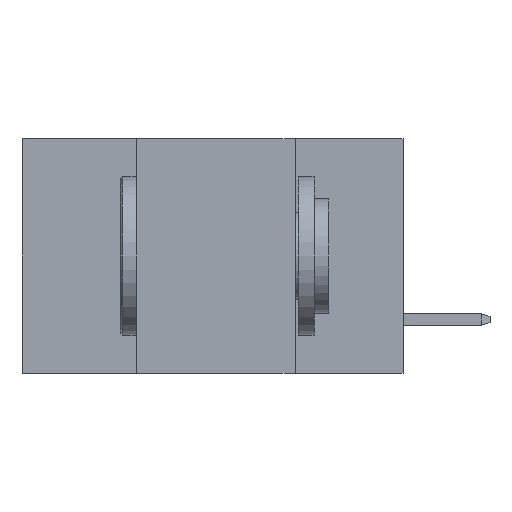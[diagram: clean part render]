
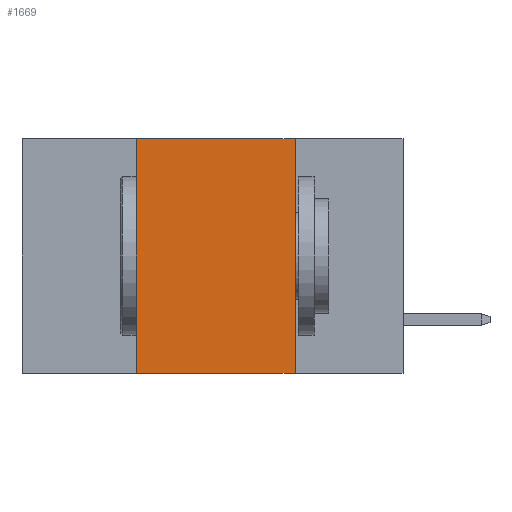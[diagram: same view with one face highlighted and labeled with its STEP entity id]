
A CAD part, left-side view. The second image highlights one B-rep face of the part: STEP entity #1669.
In plain terms, the highlighted planar face has unit normal (-1, 0, 0).
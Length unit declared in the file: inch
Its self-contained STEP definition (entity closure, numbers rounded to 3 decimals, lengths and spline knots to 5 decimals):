
#186 = AXIS2_PLACEMENT_3D ( 'NONE', #12351, #15154, #7084 ) ;
#1012 = ORIENTED_EDGE ( 'NONE', *, *, #2403, .F. ) ;
#1111 = EDGE_LOOP ( 'NONE', ( #17366, #12886, #1012, #2342 ) ) ;
#1669 = ADVANCED_FACE ( 'NONE', ( #16568 ), #1722, .F. ) ;
#1722 = PLANE ( 'NONE',  #186 ) ;
#1802 = CARTESIAN_POINT ( 'NONE',  ( 0., 0.42, 0. ) ) ;
#2342 = ORIENTED_EDGE ( 'NONE', *, *, #7177, .T. ) ;
#2403 = EDGE_CURVE ( 'NONE', #5977, #9764, #13399, .T. ) ;
#2577 = DIRECTION ( 'NONE',  ( 0., -1., 0. ) ) ;
#3229 = LINE ( 'NONE', #7332, #10016 ) ;
#3397 = VECTOR ( 'NONE', #6718, 39.37008 ) ;
#5225 = EDGE_CURVE ( 'NONE', #9764, #9868, #12114, .T. ) ;
#5361 = LINE ( 'NONE', #14443, #3397 ) ;
#5977 = VERTEX_POINT ( 'NONE', #16443 ) ;
#6151 = EDGE_CURVE ( 'NONE', #9868, #8075, #3229, .T. ) ;
#6718 = DIRECTION ( 'NONE',  ( 0., -1., 0. ) ) ;
#7084 = DIRECTION ( 'NONE',  ( 0., 0., -1. ) ) ;
#7177 = EDGE_CURVE ( 'NONE', #5977, #8075, #5361, .T. ) ;
#7332 = CARTESIAN_POINT ( 'NONE',  ( 0., 0.17, 0. ) ) ;
#7426 = DIRECTION ( 'NONE',  ( 0., 0., -1. ) ) ;
#7980 = VECTOR ( 'NONE', #2577, 39.37008 ) ;
#8075 = VERTEX_POINT ( 'NONE', #14685 ) ;
#9077 = CARTESIAN_POINT ( 'NONE',  ( 0., 0.17, 0. ) ) ;
#9764 = VERTEX_POINT ( 'NONE', #1802 ) ;
#9868 = VERTEX_POINT ( 'NONE', #9077 ) ;
#10016 = VECTOR ( 'NONE', #7426, 39.37008 ) ;
#12040 = VECTOR ( 'NONE', #13313, 39.37008 ) ;
#12114 = LINE ( 'NONE', #12391, #7980 ) ;
#12351 = CARTESIAN_POINT ( 'NONE',  ( 0., 0.6, 0. ) ) ;
#12391 = CARTESIAN_POINT ( 'NONE',  ( 0., 0.6, 0. ) ) ;
#12886 = ORIENTED_EDGE ( 'NONE', *, *, #5225, .F. ) ;
#13313 = DIRECTION ( 'NONE',  ( 0., 0., 1. ) ) ;
#13399 = LINE ( 'NONE', #14490, #12040 ) ;
#14443 = CARTESIAN_POINT ( 'NONE',  ( 0., 0.6, -0.37 ) ) ;
#14490 = CARTESIAN_POINT ( 'NONE',  ( 0., 0.42, 0. ) ) ;
#14685 = CARTESIAN_POINT ( 'NONE',  ( 0., 0.17, -0.37 ) ) ;
#15154 = DIRECTION ( 'NONE',  ( 1., 0., 0. ) ) ;
#16443 = CARTESIAN_POINT ( 'NONE',  ( 0., 0.42, -0.37 ) ) ;
#16568 = FACE_OUTER_BOUND ( 'NONE', #1111, .T. ) ;
#17366 = ORIENTED_EDGE ( 'NONE', *, *, #6151, .F. ) ;
